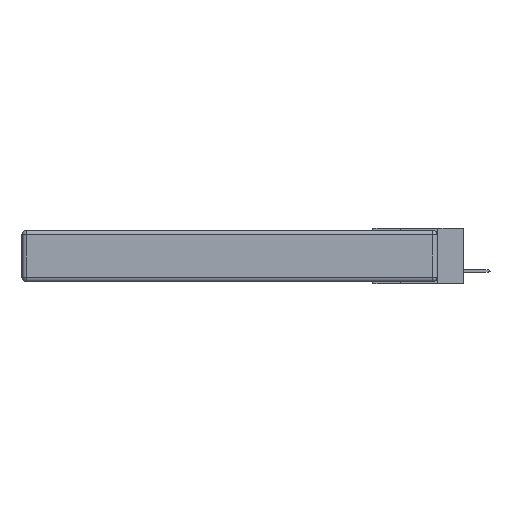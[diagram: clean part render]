
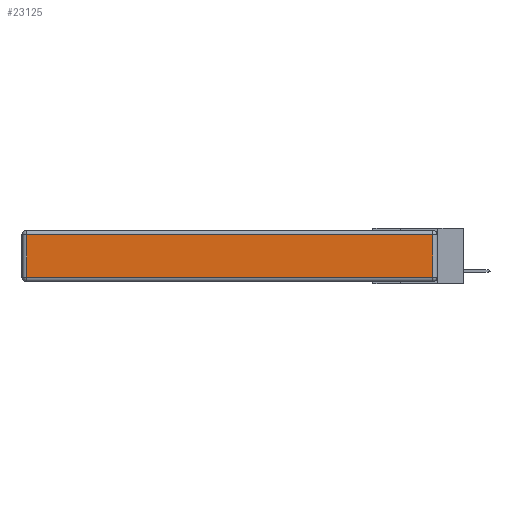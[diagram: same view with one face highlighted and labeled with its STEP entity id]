
A CAD part, left-side view. The second image highlights one B-rep face of the part: STEP entity #23125.
In plain terms, the highlighted planar face has unit normal (-1, 0, 0).
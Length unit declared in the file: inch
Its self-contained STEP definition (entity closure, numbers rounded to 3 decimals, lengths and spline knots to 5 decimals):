
#2031 = DIRECTION ( 'NONE',  ( 0., 0., 1. ) ) ;
#2283 = AXIS2_PLACEMENT_3D ( 'NONE', #9196, #25969, #21482 ) ;
#4768 = VECTOR ( 'NONE', #9171, 39.37008 ) ;
#4837 = LINE ( 'NONE', #24661, #19137 ) ;
#5334 = CARTESIAN_POINT ( 'NONE',  ( 0., 2.72, -0.03 ) ) ;
#5340 = CARTESIAN_POINT ( 'NONE',  ( 0., 0., -0.313 ) ) ;
#6483 = ORIENTED_EDGE ( 'NONE', *, *, #20835, .T. ) ;
#6619 = CARTESIAN_POINT ( 'NONE',  ( 0., 0.03, -0.03 ) ) ;
#8830 = EDGE_CURVE ( 'NONE', #21699, #29145, #4837, .T. ) ;
#9171 = DIRECTION ( 'NONE',  ( 0., 1., 0. ) ) ;
#9196 = CARTESIAN_POINT ( 'NONE',  ( 0., 0., -0.343 ) ) ;
#11193 = LINE ( 'NONE', #5340, #26963 ) ;
#12029 = VERTEX_POINT ( 'NONE', #23218 ) ;
#12754 = EDGE_CURVE ( 'NONE', #12029, #16843, #20481, .T. ) ;
#13878 = CARTESIAN_POINT ( 'NONE',  ( 0., 0.03, -0.343 ) ) ;
#16291 = CARTESIAN_POINT ( 'NONE',  ( 0., 2.75, -0.03 ) ) ;
#16843 = VERTEX_POINT ( 'NONE', #6619 ) ;
#17102 = DIRECTION ( 'NONE',  ( 0., -1., 0. ) ) ;
#17383 = EDGE_LOOP ( 'NONE', ( #6483, #19721, #21587, #22849 ) ) ;
#17428 = FACE_OUTER_BOUND ( 'NONE', #17383, .T. ) ;
#19137 = VECTOR ( 'NONE', #24542, 39.37008 ) ;
#19721 = ORIENTED_EDGE ( 'NONE', *, *, #12754, .T. ) ;
#20481 = LINE ( 'NONE', #13878, #27606 ) ;
#20835 = EDGE_CURVE ( 'NONE', #29145, #12029, #11193, .T. ) ;
#21376 = EDGE_CURVE ( 'NONE', #16843, #21699, #23964, .T. ) ;
#21482 = DIRECTION ( 'NONE',  ( 0., 0., 1. ) ) ;
#21587 = ORIENTED_EDGE ( 'NONE', *, *, #21376, .T. ) ;
#21699 = VERTEX_POINT ( 'NONE', #5334 ) ;
#22849 = ORIENTED_EDGE ( 'NONE', *, *, #8830, .T. ) ;
#23033 = CARTESIAN_POINT ( 'NONE',  ( 0., 2.72, -0.313 ) ) ;
#23125 = ADVANCED_FACE ( 'NONE', ( #17428 ), #23510, .T. ) ;
#23218 = CARTESIAN_POINT ( 'NONE',  ( 0., 0.03, -0.313 ) ) ;
#23510 = PLANE ( 'NONE',  #2283 ) ;
#23964 = LINE ( 'NONE', #16291, #4768 ) ;
#24542 = DIRECTION ( 'NONE',  ( 0., 0., -1. ) ) ;
#24661 = CARTESIAN_POINT ( 'NONE',  ( 0., 2.72, -0.343 ) ) ;
#25969 = DIRECTION ( 'NONE',  ( -1., 0., 0. ) ) ;
#26963 = VECTOR ( 'NONE', #17102, 39.37008 ) ;
#27606 = VECTOR ( 'NONE', #2031, 39.37008 ) ;
#29145 = VERTEX_POINT ( 'NONE', #23033 ) ;
